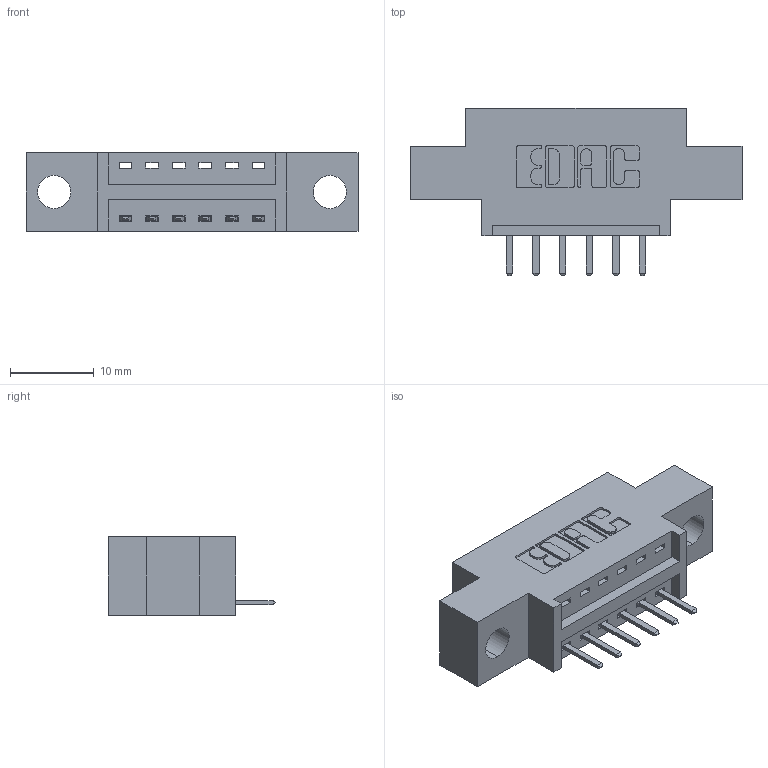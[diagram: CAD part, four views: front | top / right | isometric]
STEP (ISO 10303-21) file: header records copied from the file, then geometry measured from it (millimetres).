
FILE_DESCRIPTION (( 'STEP AP203' ), '1' );
FILE_NAME ('346-006-520-604.STEP', '2022-05-04T18:25:32', ( '' ), ( '' ), 'SwSTEP 2.0', 'SolidWorks 2020', '' );
FILE_SCHEMA (( 'CONFIG_CONTROL_DESIGN' ));
Length unit declared in the file: inch
Products named in the file (3): 346 Part_0.170 Offset - 0.156 Dia-TH; 346-006-520-604; 345-292-001_345-293-120
Assembly tree (7 placements, depth 2):
  346-006-520-604
    346 Part_0.170 Offset - 0.156 Dia-TH
    345-292-001_345-293-120  x6
Bounding box: 39.62 x 20.02 x 9.4 mm (x, y, z)
Volume: 3267 mm3; surface area: 3634.9 mm2
Topology: 7 solids, 7 shells, 512 faces, 1481 edges, 970 vertices
Faces by surface type: plane 346, cylinder 166
Entity records: 9235 total; most frequent: CARTESIAN_POINT 1616, ORIENTED_EDGE 1542, DIRECTION 1455, EDGE_CURVE 771, LINE 611, VECTOR 611, VERTEX_POINT 510, AXIS2_PLACEMENT_3D 422
